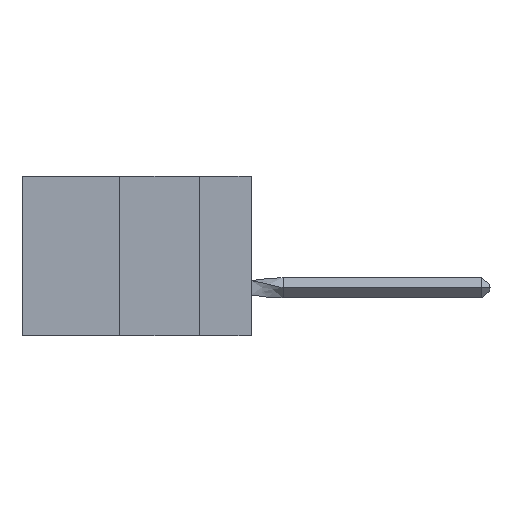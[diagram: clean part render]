
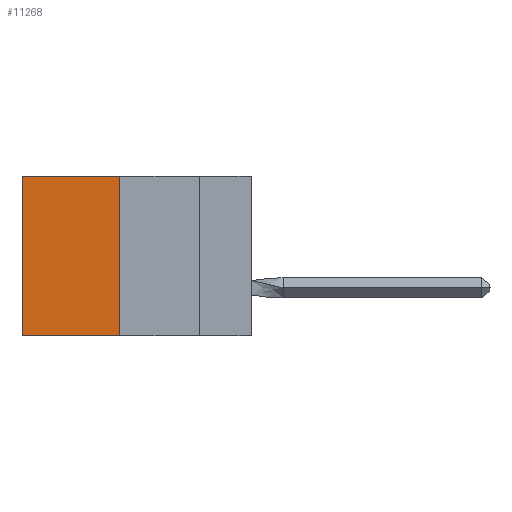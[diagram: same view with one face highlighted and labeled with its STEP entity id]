
A CAD part, left-side view. The second image highlights one B-rep face of the part: STEP entity #11268.
In plain terms, the highlighted planar face has unit normal (-1, 0, 0).
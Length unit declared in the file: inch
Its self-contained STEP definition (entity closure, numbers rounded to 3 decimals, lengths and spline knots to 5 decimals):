
#1492 = DIRECTION ( 'NONE',  ( 0., 0., -1. ) ) ;
#1833 = VERTEX_POINT ( 'NONE', #22381 ) ;
#3336 = DIRECTION ( 'NONE',  ( 1., 0., 0. ) ) ;
#3428 = DIRECTION ( 'NONE',  ( 0., 0., -1. ) ) ;
#4510 = EDGE_CURVE ( 'NONE', #13213, #14042, #14773, .T. ) ;
#5956 = VECTOR ( 'NONE', #9609, 39.37008 ) ;
#6596 = LINE ( 'NONE', #15321, #8520 ) ;
#6992 = ORIENTED_EDGE ( 'NONE', *, *, #8312, .T. ) ;
#7003 = DIRECTION ( 'NONE',  ( 0., 1., 0. ) ) ;
#7360 = DIRECTION ( 'NONE',  ( 0., 1., 0. ) ) ;
#7947 = VECTOR ( 'NONE', #7003, 39.37008 ) ;
#8312 = EDGE_CURVE ( 'NONE', #26150, #13213, #20739, .T. ) ;
#8520 = VECTOR ( 'NONE', #7360, 39.37008 ) ;
#9508 = CARTESIAN_POINT ( 'NONE',  ( 0.305, 0.72, 0. ) ) ;
#9609 = DIRECTION ( 'NONE',  ( 0., 0., -1. ) ) ;
#10871 = CARTESIAN_POINT ( 'NONE',  ( 0.305, 0.72, -0.5 ) ) ;
#11268 = ADVANCED_FACE ( 'NONE', ( #24414 ), #25795, .F. ) ;
#11508 = ORIENTED_EDGE ( 'NONE', *, *, #17536, .F. ) ;
#11628 = EDGE_LOOP ( 'NONE', ( #18564, #11508, #12753, #6992 ) ) ;
#12020 = CARTESIAN_POINT ( 'NONE',  ( 0.305, 0.413, -0.5 ) ) ;
#12753 = ORIENTED_EDGE ( 'NONE', *, *, #17565, .F. ) ;
#13213 = VERTEX_POINT ( 'NONE', #9508 ) ;
#13423 = AXIS2_PLACEMENT_3D ( 'NONE', #15623, #3336, #3428 ) ;
#14042 = VERTEX_POINT ( 'NONE', #10871 ) ;
#14773 = LINE ( 'NONE', #15999, #22165 ) ;
#15321 = CARTESIAN_POINT ( 'NONE',  ( 0.305, 0.413, -0.5 ) ) ;
#15623 = CARTESIAN_POINT ( 'NONE',  ( 0.305, 0.413, -0.5 ) ) ;
#15999 = CARTESIAN_POINT ( 'NONE',  ( 0.305, 0.72, -0.5 ) ) ;
#17536 = EDGE_CURVE ( 'NONE', #1833, #14042, #6596, .T. ) ;
#17565 = EDGE_CURVE ( 'NONE', #26150, #1833, #22923, .T. ) ;
#18564 = ORIENTED_EDGE ( 'NONE', *, *, #4510, .T. ) ;
#20739 = LINE ( 'NONE', #25491, #7947 ) ;
#22040 = CARTESIAN_POINT ( 'NONE',  ( 0.305, 0.413, 0. ) ) ;
#22165 = VECTOR ( 'NONE', #1492, 39.37008 ) ;
#22381 = CARTESIAN_POINT ( 'NONE',  ( 0.305, 0.413, -0.5 ) ) ;
#22923 = LINE ( 'NONE', #12020, #5956 ) ;
#24414 = FACE_OUTER_BOUND ( 'NONE', #11628, .T. ) ;
#25491 = CARTESIAN_POINT ( 'NONE',  ( 0.305, 0.413, 0. ) ) ;
#25795 = PLANE ( 'NONE',  #13423 ) ;
#26150 = VERTEX_POINT ( 'NONE', #22040 ) ;
